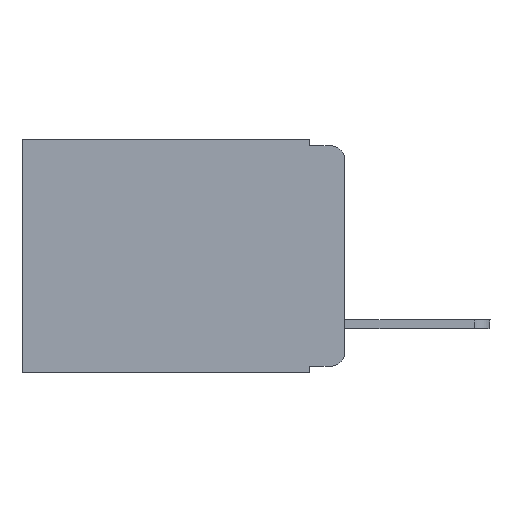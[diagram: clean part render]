
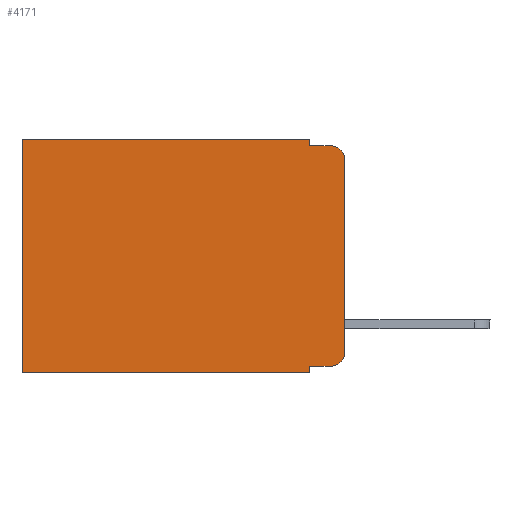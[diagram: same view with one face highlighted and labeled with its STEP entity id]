
A CAD part, left-side view. The second image highlights one B-rep face of the part: STEP entity #4171.
In plain terms, the highlighted planar face has unit normal (-1, 0, 0).
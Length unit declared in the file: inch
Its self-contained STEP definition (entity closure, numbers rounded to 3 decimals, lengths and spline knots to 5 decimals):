
#690 = LINE ( 'NONE', #5426, #17090 ) ;
#701 = EDGE_CURVE ( 'NONE', #22968, #8062, #17410, .T. ) ;
#863 = FACE_OUTER_BOUND ( 'NONE', #23650, .T. ) ;
#1064 = DIRECTION ( 'NONE',  ( 0., -1., 0. ) ) ;
#1324 = LINE ( 'NONE', #10423, #10607 ) ;
#1551 = DIRECTION ( 'NONE',  ( 0., 1., 0. ) ) ;
#1870 = ORIENTED_EDGE ( 'NONE', *, *, #23341, .T. ) ;
#1881 = EDGE_CURVE ( 'NONE', #12942, #23595, #14414, .T. ) ;
#1963 = ORIENTED_EDGE ( 'NONE', *, *, #20334, .T. ) ;
#2018 = CARTESIAN_POINT ( 'NONE',  ( 0.298, 0.02, -0.333 ) ) ;
#2098 = EDGE_CURVE ( 'NONE', #24481, #6461, #16151, .T. ) ;
#2561 = CARTESIAN_POINT ( 'NONE',  ( 0.298, 0.051, -0.343 ) ) ;
#2629 = CARTESIAN_POINT ( 'NONE',  ( 0.298, 0., 0. ) ) ;
#2790 = LINE ( 'NONE', #15416, #3100 ) ;
#2937 = DIRECTION ( 'NONE',  ( 0., 0., -1. ) ) ;
#3100 = VECTOR ( 'NONE', #4134, 39.37008 ) ;
#3263 = ORIENTED_EDGE ( 'NONE', *, *, #1881, .F. ) ;
#3439 = AXIS2_PLACEMENT_3D ( 'NONE', #14478, #5006, #2937 ) ;
#3601 = CARTESIAN_POINT ( 'NONE',  ( 0.298, 0.02, -0.03 ) ) ;
#4134 = DIRECTION ( 'NONE',  ( 0., 1., 0. ) ) ;
#4171 = ADVANCED_FACE ( 'NONE', ( #863 ), #13587, .F. ) ;
#4425 = DIRECTION ( 'NONE',  ( 0., 0., -1. ) ) ;
#4876 = ORIENTED_EDGE ( 'NONE', *, *, #701, .F. ) ;
#4904 = ORIENTED_EDGE ( 'NONE', *, *, #17049, .T. ) ;
#5006 = DIRECTION ( 'NONE',  ( -1., 0., 0. ) ) ;
#5426 = CARTESIAN_POINT ( 'NONE',  ( 0.298, 0.473, 0. ) ) ;
#5516 = DIRECTION ( 'NONE',  ( 0., 0., -1. ) ) ;
#5780 = VERTEX_POINT ( 'NONE', #15609 ) ;
#5822 = CIRCLE ( 'NONE', #3439, 0.02 ) ;
#5877 = AXIS2_PLACEMENT_3D ( 'NONE', #6285, #13746, #4425 ) ;
#6285 = CARTESIAN_POINT ( 'NONE',  ( 0.298, 0., 0. ) ) ;
#6318 = EDGE_CURVE ( 'NONE', #6461, #5780, #2790, .T. ) ;
#6368 = ORIENTED_EDGE ( 'NONE', *, *, #11425, .F. ) ;
#6461 = VERTEX_POINT ( 'NONE', #2561 ) ;
#6471 = CARTESIAN_POINT ( 'NONE',  ( 0.298, 0.051, 0. ) ) ;
#6597 = CARTESIAN_POINT ( 'NONE',  ( 0.298, 0.051, -0.01 ) ) ;
#6765 = VECTOR ( 'NONE', #16056, 39.37008 ) ;
#7943 = VERTEX_POINT ( 'NONE', #2018 ) ;
#8062 = VERTEX_POINT ( 'NONE', #13821 ) ;
#8156 = CARTESIAN_POINT ( 'NONE',  ( 0.298, 0.051, 0. ) ) ;
#8814 = CARTESIAN_POINT ( 'NONE',  ( 0.298, 0.473, 0. ) ) ;
#9610 = CARTESIAN_POINT ( 'NONE',  ( 0.298, 0., -0.03 ) ) ;
#10423 = CARTESIAN_POINT ( 'NONE',  ( 0.298, 0.051, -0.333 ) ) ;
#10544 = CARTESIAN_POINT ( 'NONE',  ( 0.298, 0., 0. ) ) ;
#10607 = VECTOR ( 'NONE', #17884, 39.37008 ) ;
#11184 = VECTOR ( 'NONE', #14678, 39.37008 ) ;
#11396 = EDGE_CURVE ( 'NONE', #7943, #8062, #5822, .T. ) ;
#11425 = EDGE_CURVE ( 'NONE', #23595, #23196, #19135, .T. ) ;
#11530 = EDGE_CURVE ( 'NONE', #14247, #5780, #690, .T. ) ;
#12942 = VERTEX_POINT ( 'NONE', #6471 ) ;
#13160 = CARTESIAN_POINT ( 'NONE',  ( 0.298, 0.051, -0.333 ) ) ;
#13587 = PLANE ( 'NONE',  #5877 ) ;
#13746 = DIRECTION ( 'NONE',  ( 1., 0., 0. ) ) ;
#13821 = CARTESIAN_POINT ( 'NONE',  ( 0.298, 0., -0.313 ) ) ;
#14247 = VERTEX_POINT ( 'NONE', #8814 ) ;
#14414 = LINE ( 'NONE', #8156, #19102 ) ;
#14478 = CARTESIAN_POINT ( 'NONE',  ( 0.298, 0.02, -0.313 ) ) ;
#14678 = DIRECTION ( 'NONE',  ( 0., 0., -1. ) ) ;
#14870 = ORIENTED_EDGE ( 'NONE', *, *, #6318, .F. ) ;
#15212 = VECTOR ( 'NONE', #1551, 39.37008 ) ;
#15250 = ORIENTED_EDGE ( 'NONE', *, *, #11396, .T. ) ;
#15416 = CARTESIAN_POINT ( 'NONE',  ( 0.298, 0., -0.343 ) ) ;
#15565 = CIRCLE ( 'NONE', #17580, 0.02 ) ;
#15609 = CARTESIAN_POINT ( 'NONE',  ( 0.298, 0.473, -0.343 ) ) ;
#16056 = DIRECTION ( 'NONE',  ( 0., 0., -1. ) ) ;
#16151 = LINE ( 'NONE', #16316, #11184 ) ;
#16316 = CARTESIAN_POINT ( 'NONE',  ( 0.298, 0.051, 0. ) ) ;
#17049 = EDGE_CURVE ( 'NONE', #24481, #7943, #1324, .T. ) ;
#17090 = VECTOR ( 'NONE', #24352, 39.37008 ) ;
#17410 = LINE ( 'NONE', #2629, #6765 ) ;
#17580 = AXIS2_PLACEMENT_3D ( 'NONE', #3601, #19072, #5516 ) ;
#17884 = DIRECTION ( 'NONE',  ( 0., -1., 0. ) ) ;
#18090 = CARTESIAN_POINT ( 'NONE',  ( 0.298, 0.02, -0.01 ) ) ;
#18252 = VECTOR ( 'NONE', #1064, 39.37008 ) ;
#19072 = DIRECTION ( 'NONE',  ( -1., 0., 0. ) ) ;
#19102 = VECTOR ( 'NONE', #19613, 39.37008 ) ;
#19135 = LINE ( 'NONE', #23682, #18252 ) ;
#19613 = DIRECTION ( 'NONE',  ( 0., 0., -1. ) ) ;
#20009 = ORIENTED_EDGE ( 'NONE', *, *, #11530, .T. ) ;
#20334 = EDGE_CURVE ( 'NONE', #12942, #14247, #22320, .T. ) ;
#22320 = LINE ( 'NONE', #10544, #15212 ) ;
#22968 = VERTEX_POINT ( 'NONE', #9610 ) ;
#23196 = VERTEX_POINT ( 'NONE', #18090 ) ;
#23341 = EDGE_CURVE ( 'NONE', #22968, #23196, #15565, .T. ) ;
#23595 = VERTEX_POINT ( 'NONE', #6597 ) ;
#23650 = EDGE_LOOP ( 'NONE', ( #4876, #1870, #6368, #3263, #1963, #20009, #14870, #24244, #4904, #15250 ) ) ;
#23682 = CARTESIAN_POINT ( 'NONE',  ( 0.298, 0.051, -0.01 ) ) ;
#24244 = ORIENTED_EDGE ( 'NONE', *, *, #2098, .F. ) ;
#24352 = DIRECTION ( 'NONE',  ( 0., 0., -1. ) ) ;
#24481 = VERTEX_POINT ( 'NONE', #13160 ) ;
